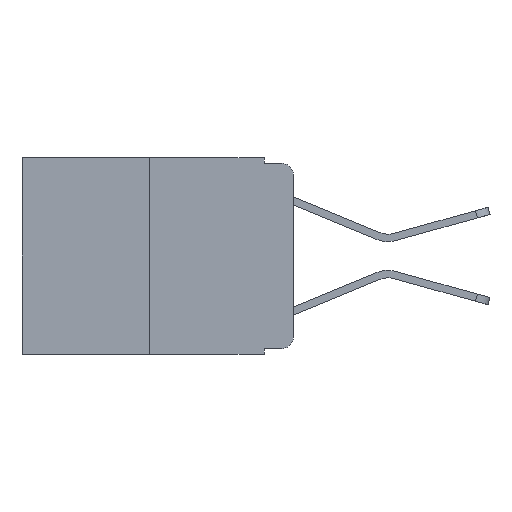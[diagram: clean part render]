
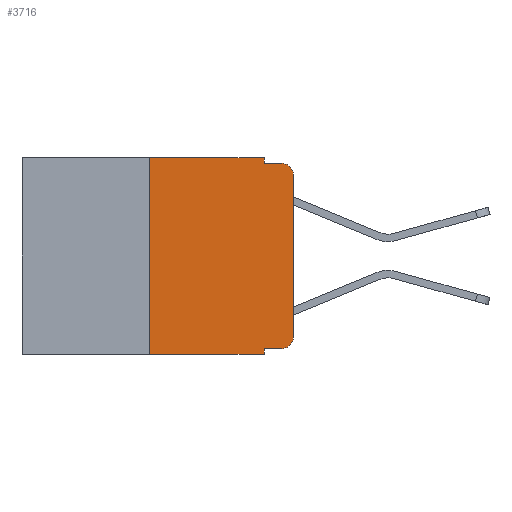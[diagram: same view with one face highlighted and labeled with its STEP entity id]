
A CAD part, left-side view. The second image highlights one B-rep face of the part: STEP entity #3716.
In plain terms, the highlighted planar face has unit normal (-1, 0, 0).
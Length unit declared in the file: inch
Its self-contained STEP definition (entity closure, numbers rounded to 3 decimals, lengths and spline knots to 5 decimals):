
#60 = DIRECTION ( 'NONE',  ( 0., 0., -1. ) ) ;
#209 = EDGE_CURVE ( 'NONE', #9636, #8667, #10788, .T. ) ;
#485 = LINE ( 'NONE', #12871, #11073 ) ;
#583 = DIRECTION ( 'NONE',  ( 0., 0., -1. ) ) ;
#779 = ORIENTED_EDGE ( 'NONE', *, *, #7428, .F. ) ;
#850 = CARTESIAN_POINT ( 'NONE',  ( 0., 0.051, -0.343 ) ) ;
#857 = CARTESIAN_POINT ( 'NONE',  ( 0., 0.02, -0.313 ) ) ;
#864 = DIRECTION ( 'NONE',  ( 0., 0., 1. ) ) ;
#923 = CARTESIAN_POINT ( 'NONE',  ( 0., 0.25, -0.343 ) ) ;
#1328 = CIRCLE ( 'NONE', #6712, 0.02 ) ;
#1390 = PLANE ( 'NONE',  #9481 ) ;
#1492 = VERTEX_POINT ( 'NONE', #923 ) ;
#1806 = FACE_OUTER_BOUND ( 'NONE', #4637, .T. ) ;
#1956 = DIRECTION ( 'NONE',  ( 0., 0., -1. ) ) ;
#2132 = VECTOR ( 'NONE', #2303, 39.37008 ) ;
#2303 = DIRECTION ( 'NONE',  ( 0., 0., -1. ) ) ;
#2918 = VERTEX_POINT ( 'NONE', #8265 ) ;
#3046 = VECTOR ( 'NONE', #8937, 39.37008 ) ;
#3048 = VECTOR ( 'NONE', #5047, 39.37008 ) ;
#3075 = ORIENTED_EDGE ( 'NONE', *, *, #4749, .F. ) ;
#3716 = ADVANCED_FACE ( 'NONE', ( #1806 ), #1390, .F. ) ;
#4315 = LINE ( 'NONE', #8320, #9279 ) ;
#4526 = ORIENTED_EDGE ( 'NONE', *, *, #9652, .T. ) ;
#4604 = VERTEX_POINT ( 'NONE', #11310 ) ;
#4637 = EDGE_LOOP ( 'NONE', ( #10198, #10490, #10768, #3075, #11047, #779, #4526, #10043, #7834, #5801 ) ) ;
#4749 = EDGE_CURVE ( 'NONE', #8659, #9636, #8849, .T. ) ;
#4884 = VERTEX_POINT ( 'NONE', #5464 ) ;
#5047 = DIRECTION ( 'NONE',  ( 0., -1., 0. ) ) ;
#5071 = VECTOR ( 'NONE', #9581, 39.37008 ) ;
#5464 = CARTESIAN_POINT ( 'NONE',  ( 0., 0., -0.313 ) ) ;
#5604 = CARTESIAN_POINT ( 'NONE',  ( 0., 0.051, 0. ) ) ;
#5801 = ORIENTED_EDGE ( 'NONE', *, *, #11804, .T. ) ;
#5980 = VERTEX_POINT ( 'NONE', #9363 ) ;
#6050 = CARTESIAN_POINT ( 'NONE',  ( 0., 0.473, 0. ) ) ;
#6320 = VECTOR ( 'NONE', #11936, 39.37008 ) ;
#6593 = DIRECTION ( 'NONE',  ( -1., 0., 0. ) ) ;
#6636 = LINE ( 'NONE', #7286, #6320 ) ;
#6685 = CARTESIAN_POINT ( 'NONE',  ( 0., 0., 0. ) ) ;
#6712 = AXIS2_PLACEMENT_3D ( 'NONE', #12220, #6593, #60 ) ;
#7001 = EDGE_CURVE ( 'NONE', #4884, #10579, #7709, .T. ) ;
#7286 = CARTESIAN_POINT ( 'NONE',  ( 0., 0.051, -0.333 ) ) ;
#7301 = CARTESIAN_POINT ( 'NONE',  ( 0., 0.051, 0. ) ) ;
#7428 = EDGE_CURVE ( 'NONE', #1492, #5980, #485, .T. ) ;
#7709 = LINE ( 'NONE', #6685, #5071 ) ;
#7834 = ORIENTED_EDGE ( 'NONE', *, *, #10613, .T. ) ;
#8230 = CARTESIAN_POINT ( 'NONE',  ( 0., 0.02, -0.01 ) ) ;
#8240 = LINE ( 'NONE', #9891, #3048 ) ;
#8265 = CARTESIAN_POINT ( 'NONE',  ( 0., 0.02, -0.333 ) ) ;
#8295 = DIRECTION ( 'NONE',  ( -1., 0., 0. ) ) ;
#8320 = CARTESIAN_POINT ( 'NONE',  ( 0., 0.473, 0. ) ) ;
#8659 = VERTEX_POINT ( 'NONE', #7301 ) ;
#8667 = VERTEX_POINT ( 'NONE', #8230 ) ;
#8817 = DIRECTION ( 'NONE',  ( 1., 0., 0. ) ) ;
#8849 = LINE ( 'NONE', #8972, #3046 ) ;
#8937 = DIRECTION ( 'NONE',  ( 0., 0., -1. ) ) ;
#8972 = CARTESIAN_POINT ( 'NONE',  ( 0., 0.051, 0. ) ) ;
#9250 = CARTESIAN_POINT ( 'NONE',  ( 0., 0.051, -0.01 ) ) ;
#9266 = DIRECTION ( 'NONE',  ( 0., -1., 0. ) ) ;
#9279 = VECTOR ( 'NONE', #9266, 39.37008 ) ;
#9363 = CARTESIAN_POINT ( 'NONE',  ( 0., 0.25, 0. ) ) ;
#9481 = AXIS2_PLACEMENT_3D ( 'NONE', #6050, #8817, #583 ) ;
#9581 = DIRECTION ( 'NONE',  ( 0., 0., 1. ) ) ;
#9636 = VERTEX_POINT ( 'NONE', #12573 ) ;
#9652 = EDGE_CURVE ( 'NONE', #1492, #11429, #8240, .T. ) ;
#9767 = DIRECTION ( 'NONE',  ( 0., -1., 0. ) ) ;
#9793 = EDGE_CURVE ( 'NONE', #5980, #8659, #4315, .T. ) ;
#9891 = CARTESIAN_POINT ( 'NONE',  ( 0., 0.473, -0.343 ) ) ;
#9982 = EDGE_CURVE ( 'NONE', #4604, #11429, #12696, .T. ) ;
#10043 = ORIENTED_EDGE ( 'NONE', *, *, #9982, .F. ) ;
#10198 = ORIENTED_EDGE ( 'NONE', *, *, #7001, .T. ) ;
#10334 = AXIS2_PLACEMENT_3D ( 'NONE', #857, #8295, #1956 ) ;
#10490 = ORIENTED_EDGE ( 'NONE', *, *, #10832, .T. ) ;
#10512 = VECTOR ( 'NONE', #9767, 39.37008 ) ;
#10579 = VERTEX_POINT ( 'NONE', #12801 ) ;
#10613 = EDGE_CURVE ( 'NONE', #4604, #2918, #6636, .T. ) ;
#10768 = ORIENTED_EDGE ( 'NONE', *, *, #209, .F. ) ;
#10788 = LINE ( 'NONE', #9250, #10512 ) ;
#10832 = EDGE_CURVE ( 'NONE', #10579, #8667, #1328, .T. ) ;
#11047 = ORIENTED_EDGE ( 'NONE', *, *, #9793, .F. ) ;
#11073 = VECTOR ( 'NONE', #864, 39.37008 ) ;
#11310 = CARTESIAN_POINT ( 'NONE',  ( 0., 0.051, -0.333 ) ) ;
#11429 = VERTEX_POINT ( 'NONE', #850 ) ;
#11804 = EDGE_CURVE ( 'NONE', #2918, #4884, #12319, .T. ) ;
#11936 = DIRECTION ( 'NONE',  ( 0., -1., 0. ) ) ;
#12220 = CARTESIAN_POINT ( 'NONE',  ( 0., 0.02, -0.03 ) ) ;
#12319 = CIRCLE ( 'NONE', #10334, 0.02 ) ;
#12573 = CARTESIAN_POINT ( 'NONE',  ( 0., 0.051, -0.01 ) ) ;
#12696 = LINE ( 'NONE', #5604, #2132 ) ;
#12801 = CARTESIAN_POINT ( 'NONE',  ( 0., 0., -0.03 ) ) ;
#12871 = CARTESIAN_POINT ( 'NONE',  ( 0., 0.25, 0. ) ) ;
